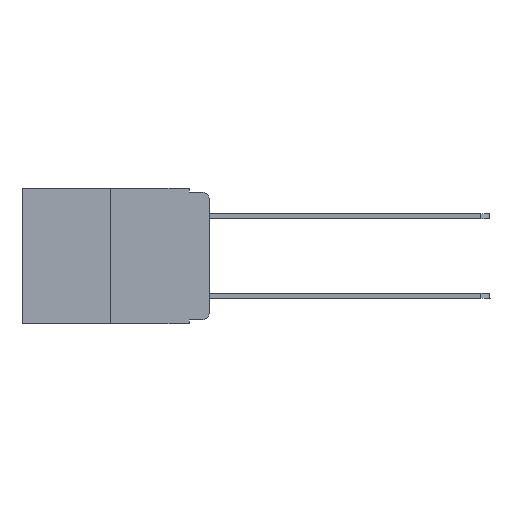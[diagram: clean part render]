
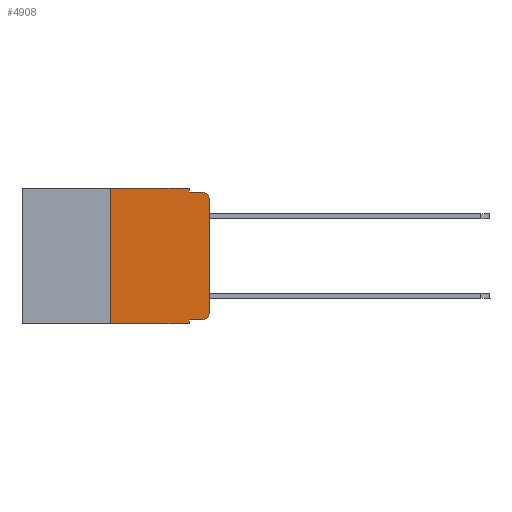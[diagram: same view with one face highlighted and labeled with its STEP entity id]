
A CAD part, left-side view. The second image highlights one B-rep face of the part: STEP entity #4908.
In plain terms, the highlighted planar face has unit normal (-1, 0, 0).
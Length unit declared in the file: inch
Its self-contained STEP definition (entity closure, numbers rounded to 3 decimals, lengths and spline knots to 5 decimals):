
#273 = ORIENTED_EDGE ( 'NONE', *, *, #342, .T. ) ;
#342 = EDGE_CURVE ( 'NONE', #13007, #3170, #5285, .T. ) ;
#636 = VERTEX_POINT ( 'NONE', #15196 ) ;
#769 = VECTOR ( 'NONE', #7561, 39.37008 ) ;
#777 = EDGE_CURVE ( 'NONE', #4944, #3610, #1519, .T. ) ;
#1135 = CARTESIAN_POINT ( 'NONE',  ( 0., 0.051, -0.01 ) ) ;
#1166 = ORIENTED_EDGE ( 'NONE', *, *, #4941, .T. ) ;
#1519 = LINE ( 'NONE', #4313, #9413 ) ;
#1648 = VERTEX_POINT ( 'NONE', #11250 ) ;
#2068 = ORIENTED_EDGE ( 'NONE', *, *, #777, .T. ) ;
#2340 = DIRECTION ( 'NONE',  ( 0., -1., 0. ) ) ;
#2524 = VECTOR ( 'NONE', #4935, 39.37008 ) ;
#2686 = EDGE_CURVE ( 'NONE', #11455, #1648, #12517, .T. ) ;
#2736 = DIRECTION ( 'NONE',  ( 1., 0., 0. ) ) ;
#3170 = VERTEX_POINT ( 'NONE', #6483 ) ;
#3339 = CARTESIAN_POINT ( 'NONE',  ( 0., 0.051, 0. ) ) ;
#3443 = DIRECTION ( 'NONE',  ( 0., -1., 0. ) ) ;
#3544 = VECTOR ( 'NONE', #6461, 39.37008 ) ;
#3610 = VERTEX_POINT ( 'NONE', #8832 ) ;
#3681 = CARTESIAN_POINT ( 'NONE',  ( 0., 0., -0.03 ) ) ;
#3810 = PLANE ( 'NONE',  #7078 ) ;
#3822 = ORIENTED_EDGE ( 'NONE', *, *, #10664, .T. ) ;
#3861 = CARTESIAN_POINT ( 'NONE',  ( 0., 0.25, -0.343 ) ) ;
#4313 = CARTESIAN_POINT ( 'NONE',  ( 0., 0.473, -0.343 ) ) ;
#4531 = DIRECTION ( 'NONE',  ( -1., 0., 0. ) ) ;
#4552 = CARTESIAN_POINT ( 'NONE',  ( 0., 0.051, 0. ) ) ;
#4674 = VECTOR ( 'NONE', #3443, 39.37008 ) ;
#4908 = ADVANCED_FACE ( 'NONE', ( #6290 ), #3810, .F. ) ;
#4935 = DIRECTION ( 'NONE',  ( 0., 0., -1. ) ) ;
#4941 = EDGE_CURVE ( 'NONE', #3170, #12273, #12450, .T. ) ;
#4944 = VERTEX_POINT ( 'NONE', #3861 ) ;
#5285 = CIRCLE ( 'NONE', #8149, 0.02 ) ;
#5322 = CIRCLE ( 'NONE', #15466, 0.02 ) ;
#5440 = VERTEX_POINT ( 'NONE', #10687 ) ;
#5466 = ORIENTED_EDGE ( 'NONE', *, *, #13640, .F. ) ;
#5670 = DIRECTION ( 'NONE',  ( -1., 0., 0. ) ) ;
#5742 = ORIENTED_EDGE ( 'NONE', *, *, #8495, .T. ) ;
#5935 = ORIENTED_EDGE ( 'NONE', *, *, #15146, .F. ) ;
#6204 = LINE ( 'NONE', #10397, #3544 ) ;
#6266 = ORIENTED_EDGE ( 'NONE', *, *, #2686, .F. ) ;
#6290 = FACE_OUTER_BOUND ( 'NONE', #11742, .T. ) ;
#6342 = EDGE_CURVE ( 'NONE', #5440, #3610, #14906, .T. ) ;
#6377 = VERTEX_POINT ( 'NONE', #4552 ) ;
#6461 = DIRECTION ( 'NONE',  ( 0., 0., 1. ) ) ;
#6483 = CARTESIAN_POINT ( 'NONE',  ( 0., 0., -0.313 ) ) ;
#7078 = AXIS2_PLACEMENT_3D ( 'NONE', #9937, #2736, #12392 ) ;
#7278 = CARTESIAN_POINT ( 'NONE',  ( 0., 0.051, -0.333 ) ) ;
#7561 = DIRECTION ( 'NONE',  ( 0., 0., 1. ) ) ;
#8139 = DIRECTION ( 'NONE',  ( 0., 0., -1. ) ) ;
#8149 = AXIS2_PLACEMENT_3D ( 'NONE', #8291, #4531, #13134 ) ;
#8291 = CARTESIAN_POINT ( 'NONE',  ( 0., 0.02, -0.313 ) ) ;
#8379 = CARTESIAN_POINT ( 'NONE',  ( 0., 0.051, -0.01 ) ) ;
#8495 = EDGE_CURVE ( 'NONE', #5440, #13007, #14255, .T. ) ;
#8679 = CARTESIAN_POINT ( 'NONE',  ( 0., 0.051, 0. ) ) ;
#8832 = CARTESIAN_POINT ( 'NONE',  ( 0., 0.051, -0.343 ) ) ;
#9044 = VECTOR ( 'NONE', #10510, 39.37008 ) ;
#9332 = EDGE_CURVE ( 'NONE', #636, #6377, #12120, .T. ) ;
#9380 = DIRECTION ( 'NONE',  ( 0., -1., 0. ) ) ;
#9413 = VECTOR ( 'NONE', #9380, 39.37008 ) ;
#9434 = CARTESIAN_POINT ( 'NONE',  ( 0., 0.02, -0.03 ) ) ;
#9937 = CARTESIAN_POINT ( 'NONE',  ( 0., 0.473, 0. ) ) ;
#10097 = VECTOR ( 'NONE', #15674, 39.37008 ) ;
#10123 = ORIENTED_EDGE ( 'NONE', *, *, #9332, .F. ) ;
#10397 = CARTESIAN_POINT ( 'NONE',  ( 0., 0.25, 0. ) ) ;
#10510 = DIRECTION ( 'NONE',  ( 0., -1., 0. ) ) ;
#10664 = EDGE_CURVE ( 'NONE', #12273, #1648, #5322, .T. ) ;
#10687 = CARTESIAN_POINT ( 'NONE',  ( 0., 0.051, -0.333 ) ) ;
#10957 = CARTESIAN_POINT ( 'NONE',  ( 0., 0.473, 0. ) ) ;
#11250 = CARTESIAN_POINT ( 'NONE',  ( 0., 0.02, -0.01 ) ) ;
#11455 = VERTEX_POINT ( 'NONE', #8379 ) ;
#11742 = EDGE_LOOP ( 'NONE', ( #1166, #3822, #6266, #5935, #10123, #5466, #2068, #13215, #5742, #273 ) ) ;
#12120 = LINE ( 'NONE', #10957, #15763 ) ;
#12273 = VERTEX_POINT ( 'NONE', #3681 ) ;
#12392 = DIRECTION ( 'NONE',  ( 0., 0., -1. ) ) ;
#12450 = LINE ( 'NONE', #14924, #769 ) ;
#12517 = LINE ( 'NONE', #1135, #4674 ) ;
#13007 = VERTEX_POINT ( 'NONE', #13093 ) ;
#13093 = CARTESIAN_POINT ( 'NONE',  ( 0., 0.02, -0.333 ) ) ;
#13134 = DIRECTION ( 'NONE',  ( 0., 0., -1. ) ) ;
#13215 = ORIENTED_EDGE ( 'NONE', *, *, #6342, .F. ) ;
#13640 = EDGE_CURVE ( 'NONE', #4944, #636, #6204, .T. ) ;
#14250 = LINE ( 'NONE', #8679, #2524 ) ;
#14255 = LINE ( 'NONE', #7278, #9044 ) ;
#14906 = LINE ( 'NONE', #3339, #10097 ) ;
#14924 = CARTESIAN_POINT ( 'NONE',  ( 0., 0., 0. ) ) ;
#15146 = EDGE_CURVE ( 'NONE', #6377, #11455, #14250, .T. ) ;
#15196 = CARTESIAN_POINT ( 'NONE',  ( 0., 0.25, 0. ) ) ;
#15466 = AXIS2_PLACEMENT_3D ( 'NONE', #9434, #5670, #8139 ) ;
#15674 = DIRECTION ( 'NONE',  ( 0., 0., -1. ) ) ;
#15763 = VECTOR ( 'NONE', #2340, 39.37008 ) ;
